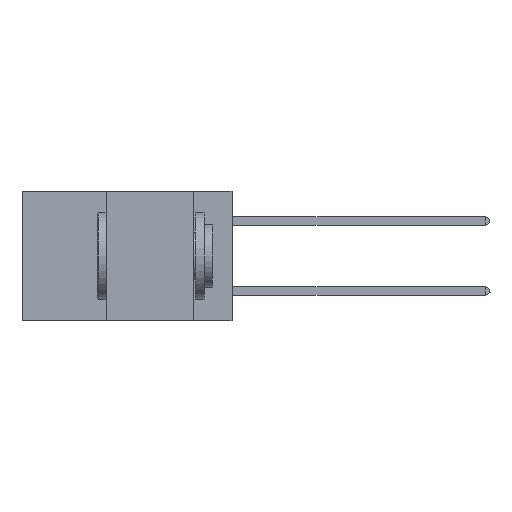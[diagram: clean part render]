
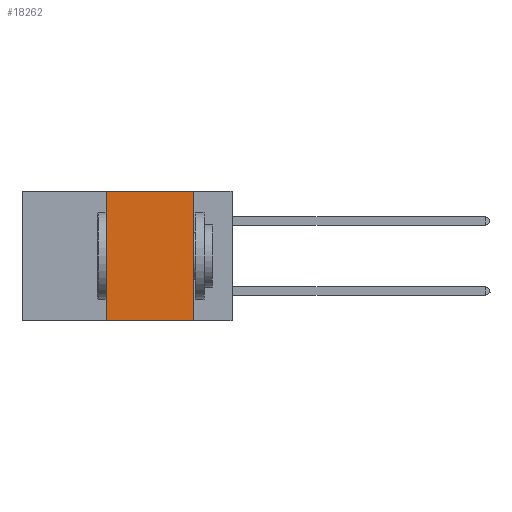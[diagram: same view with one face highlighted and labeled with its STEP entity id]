
A CAD part, left-side view. The second image highlights one B-rep face of the part: STEP entity #18262.
In plain terms, the highlighted planar face has unit normal (-1, 0, 0).
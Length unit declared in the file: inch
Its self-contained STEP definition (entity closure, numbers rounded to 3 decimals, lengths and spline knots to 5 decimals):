
#1328 = VECTOR ( 'NONE', #11228, 39.37008 ) ;
#1370 = LINE ( 'NONE', #21212, #1873 ) ;
#1873 = VECTOR ( 'NONE', #17946, 39.37008 ) ;
#2894 = LINE ( 'NONE', #4172, #7283 ) ;
#2917 = EDGE_LOOP ( 'NONE', ( #3914, #18169, #4706, #4412 ) ) ;
#2988 = VERTEX_POINT ( 'NONE', #7542 ) ;
#3648 = VECTOR ( 'NONE', #17628, 39.37008 ) ;
#3914 = ORIENTED_EDGE ( 'NONE', *, *, #8157, .F. ) ;
#4172 = CARTESIAN_POINT ( 'NONE',  ( 0., 0.36, 0. ) ) ;
#4412 = ORIENTED_EDGE ( 'NONE', *, *, #8832, .T. ) ;
#4616 = CARTESIAN_POINT ( 'NONE',  ( 0., 0.36, -0.37 ) ) ;
#4706 = ORIENTED_EDGE ( 'NONE', *, *, #8746, .F. ) ;
#5015 = CARTESIAN_POINT ( 'NONE',  ( 0., 0.6, 0. ) ) ;
#6093 = CARTESIAN_POINT ( 'NONE',  ( 0., 0.6, -0.37 ) ) ;
#6575 = CARTESIAN_POINT ( 'NONE',  ( 0., 0.11, -0.37 ) ) ;
#7283 = VECTOR ( 'NONE', #8900, 39.37008 ) ;
#7542 = CARTESIAN_POINT ( 'NONE',  ( 0., 0.11, 0. ) ) ;
#8157 = EDGE_CURVE ( 'NONE', #2988, #17814, #1370, .T. ) ;
#8746 = EDGE_CURVE ( 'NONE', #13672, #11102, #2894, .T. ) ;
#8832 = EDGE_CURVE ( 'NONE', #13672, #17814, #12687, .T. ) ;
#8900 = DIRECTION ( 'NONE',  ( 0., 0., 1. ) ) ;
#11102 = VERTEX_POINT ( 'NONE', #20861 ) ;
#11142 = LINE ( 'NONE', #14400, #1328 ) ;
#11228 = DIRECTION ( 'NONE',  ( 0., -1., 0. ) ) ;
#12687 = LINE ( 'NONE', #6093, #3648 ) ;
#13672 = VERTEX_POINT ( 'NONE', #4616 ) ;
#14400 = CARTESIAN_POINT ( 'NONE',  ( 0., 0.6, 0. ) ) ;
#17628 = DIRECTION ( 'NONE',  ( 0., -1., 0. ) ) ;
#17814 = VERTEX_POINT ( 'NONE', #6575 ) ;
#17946 = DIRECTION ( 'NONE',  ( 0., 0., -1. ) ) ;
#18169 = ORIENTED_EDGE ( 'NONE', *, *, #20376, .F. ) ;
#18238 = DIRECTION ( 'NONE',  ( 0., 0., -1. ) ) ;
#18262 = ADVANCED_FACE ( 'NONE', ( #20552 ), #19838, .F. ) ;
#19772 = DIRECTION ( 'NONE',  ( 1., 0., 0. ) ) ;
#19838 = PLANE ( 'NONE',  #21097 ) ;
#20376 = EDGE_CURVE ( 'NONE', #11102, #2988, #11142, .T. ) ;
#20552 = FACE_OUTER_BOUND ( 'NONE', #2917, .T. ) ;
#20861 = CARTESIAN_POINT ( 'NONE',  ( 0., 0.36, 0. ) ) ;
#21097 = AXIS2_PLACEMENT_3D ( 'NONE', #5015, #19772, #18238 ) ;
#21212 = CARTESIAN_POINT ( 'NONE',  ( 0., 0.11, 0. ) ) ;
